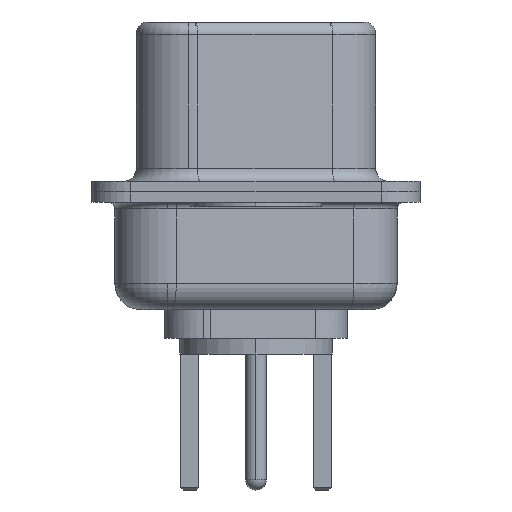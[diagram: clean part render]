
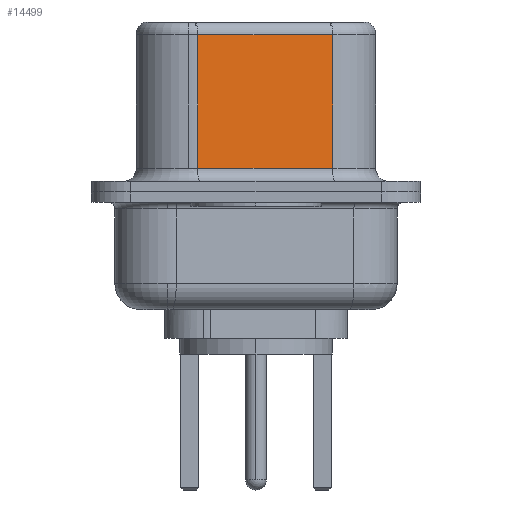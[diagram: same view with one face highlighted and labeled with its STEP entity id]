
A CAD part, left-side view. The second image highlights one B-rep face of the part: STEP entity #14499.
In plain terms, the highlighted planar face has unit normal (-0.985, -0.174, 0).
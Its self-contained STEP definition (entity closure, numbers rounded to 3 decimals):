
#274 = VERTEX_POINT ( 'NONE', #9348 ) ;
#1095 = DIRECTION ( 'NONE',  ( -0.174, 0.985, 0. ) ) ;
#1158 = LINE ( 'NONE', #9607, #4402 ) ;
#1190 = DIRECTION ( 'NONE',  ( 0.985, 0.174, 0. ) ) ;
#1392 = VERTEX_POINT ( 'NONE', #3412 ) ;
#2052 = ORIENTED_EDGE ( 'NONE', *, *, #4838, .F. ) ;
#3148 = VECTOR ( 'NONE', #1095, 1000. ) ;
#3412 = CARTESIAN_POINT ( 'NONE',  ( 3.67, 2.233, 6.02 ) ) ;
#3585 = ORIENTED_EDGE ( 'NONE', *, *, #14713, .T. ) ;
#3644 = VECTOR ( 'NONE', #9478, 1000. ) ;
#4402 = VECTOR ( 'NONE', #14179, 1000. ) ;
#4838 = EDGE_CURVE ( 'NONE', #274, #15898, #1158, .T. ) ;
#4952 = EDGE_CURVE ( 'NONE', #274, #1392, #8637, .T. ) ;
#6870 = CARTESIAN_POINT ( 'NONE',  ( 3.67, 2.233, 6.52 ) ) ;
#7497 = CARTESIAN_POINT ( 'NONE',  ( 3.67, 2.233, 0.9 ) ) ;
#8637 = LINE ( 'NONE', #8835, #3148 ) ;
#8747 = VECTOR ( 'NONE', #10092, 1000. ) ;
#8835 = CARTESIAN_POINT ( 'NONE',  ( 4.58, -2.927, 6.02 ) ) ;
#9165 = CARTESIAN_POINT ( 'NONE',  ( 4.58, -2.927, 0.9 ) ) ;
#9348 = CARTESIAN_POINT ( 'NONE',  ( 4.58, -2.927, 6.02 ) ) ;
#9478 = DIRECTION ( 'NONE',  ( 0., 0., -1. ) ) ;
#9607 = CARTESIAN_POINT ( 'NONE',  ( 4.58, -2.927, 6.52 ) ) ;
#10092 = DIRECTION ( 'NONE',  ( 0.174, -0.985, 0. ) ) ;
#10218 = ORIENTED_EDGE ( 'NONE', *, *, #4952, .T. ) ;
#10971 = AXIS2_PLACEMENT_3D ( 'NONE', #11494, #1190, #11549 ) ;
#11494 = CARTESIAN_POINT ( 'NONE',  ( 4.58, -2.927, 6.52 ) ) ;
#11549 = DIRECTION ( 'NONE',  ( -0.174, 0.985, 0. ) ) ;
#12593 = EDGE_CURVE ( 'NONE', #13094, #15898, #15254, .T. ) ;
#13094 = VERTEX_POINT ( 'NONE', #7497 ) ;
#14179 = DIRECTION ( 'NONE',  ( 0., 0., -1. ) ) ;
#14214 = FACE_OUTER_BOUND ( 'NONE', #15928, .T. ) ;
#14242 = PLANE ( 'NONE',  #10971 ) ;
#14499 = ADVANCED_FACE ( 'NONE', ( #14214 ), #14242, .F. ) ;
#14713 = EDGE_CURVE ( 'NONE', #1392, #13094, #14815, .T. ) ;
#14815 = LINE ( 'NONE', #6870, #3644 ) ;
#15254 = LINE ( 'NONE', #16352, #8747 ) ;
#15311 = ORIENTED_EDGE ( 'NONE', *, *, #12593, .T. ) ;
#15898 = VERTEX_POINT ( 'NONE', #9165 ) ;
#15928 = EDGE_LOOP ( 'NONE', ( #2052, #10218, #3585, #15311 ) ) ;
#16352 = CARTESIAN_POINT ( 'NONE',  ( 4.58, -2.927, 0.9 ) ) ;
